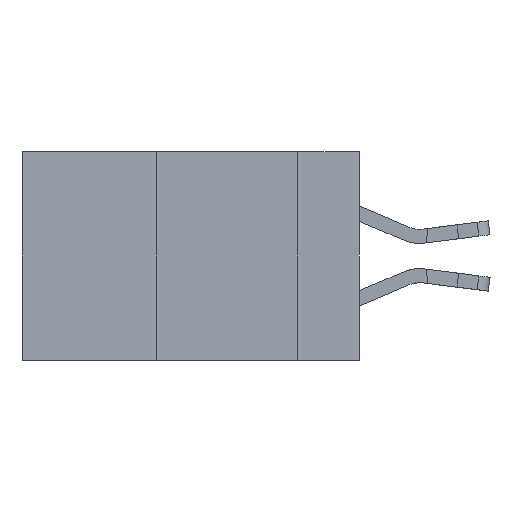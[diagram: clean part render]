
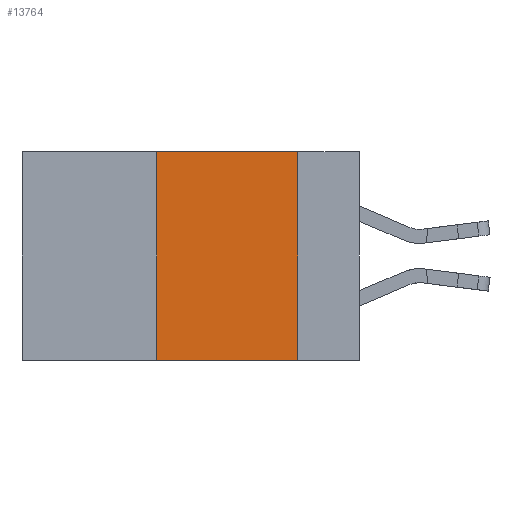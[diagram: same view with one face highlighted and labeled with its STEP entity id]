
A CAD part, left-side view. The second image highlights one B-rep face of the part: STEP entity #13764.
In plain terms, the highlighted planar face has unit normal (-1, 0, 0).
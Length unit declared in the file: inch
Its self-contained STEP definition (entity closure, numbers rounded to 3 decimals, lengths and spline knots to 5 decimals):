
#739 = EDGE_LOOP ( 'NONE', ( #3418, #4304, #5469, #11431 ) ) ;
#997 = CARTESIAN_POINT ( 'NONE',  ( 0., 0.6, 0. ) ) ;
#2953 = DIRECTION ( 'NONE',  ( 0., -1., 0. ) ) ;
#3030 = DIRECTION ( 'NONE',  ( 0., 0., -1. ) ) ;
#3277 = LINE ( 'NONE', #997, #12365 ) ;
#3418 = ORIENTED_EDGE ( 'NONE', *, *, #12719, .F. ) ;
#4304 = ORIENTED_EDGE ( 'NONE', *, *, #10136, .F. ) ;
#4345 = VECTOR ( 'NONE', #15371, 39.37008 ) ;
#4586 = FACE_OUTER_BOUND ( 'NONE', #739, .T. ) ;
#5469 = ORIENTED_EDGE ( 'NONE', *, *, #6640, .F. ) ;
#6032 = EDGE_CURVE ( 'NONE', #23045, #20653, #17434, .T. ) ;
#6603 = CARTESIAN_POINT ( 'NONE',  ( 0., 0.6, 0. ) ) ;
#6640 = EDGE_CURVE ( 'NONE', #23045, #22220, #19905, .T. ) ;
#10136 = EDGE_CURVE ( 'NONE', #22220, #14114, #3277, .T. ) ;
#10166 = AXIS2_PLACEMENT_3D ( 'NONE', #6603, #13911, #3030 ) ;
#11065 = CARTESIAN_POINT ( 'NONE',  ( 0., 0.36, -0.37 ) ) ;
#11071 = CARTESIAN_POINT ( 'NONE',  ( 0., 0.11, 0. ) ) ;
#11431 = ORIENTED_EDGE ( 'NONE', *, *, #6032, .T. ) ;
#11694 = CARTESIAN_POINT ( 'NONE',  ( 0., 0.36, 0. ) ) ;
#12365 = VECTOR ( 'NONE', #2953, 39.37008 ) ;
#12719 = EDGE_CURVE ( 'NONE', #14114, #20653, #13385, .T. ) ;
#12908 = DIRECTION ( 'NONE',  ( 0., 0., -1. ) ) ;
#13385 = LINE ( 'NONE', #11071, #22286 ) ;
#13764 = ADVANCED_FACE ( 'NONE', ( #4586 ), #22780, .F. ) ;
#13911 = DIRECTION ( 'NONE',  ( 1., 0., 0. ) ) ;
#14114 = VERTEX_POINT ( 'NONE', #22369 ) ;
#15371 = DIRECTION ( 'NONE',  ( 0., 0., 1. ) ) ;
#15499 = CARTESIAN_POINT ( 'NONE',  ( 0., 0.36, 0. ) ) ;
#16220 = DIRECTION ( 'NONE',  ( 0., -1., 0. ) ) ;
#17434 = LINE ( 'NONE', #21449, #21543 ) ;
#19905 = LINE ( 'NONE', #11694, #4345 ) ;
#20653 = VERTEX_POINT ( 'NONE', #20855 ) ;
#20855 = CARTESIAN_POINT ( 'NONE',  ( 0., 0.11, -0.37 ) ) ;
#21449 = CARTESIAN_POINT ( 'NONE',  ( 0., 0.6, -0.37 ) ) ;
#21543 = VECTOR ( 'NONE', #16220, 39.37008 ) ;
#22220 = VERTEX_POINT ( 'NONE', #15499 ) ;
#22286 = VECTOR ( 'NONE', #12908, 39.37008 ) ;
#22369 = CARTESIAN_POINT ( 'NONE',  ( 0., 0.11, 0. ) ) ;
#22780 = PLANE ( 'NONE',  #10166 ) ;
#23045 = VERTEX_POINT ( 'NONE', #11065 ) ;
